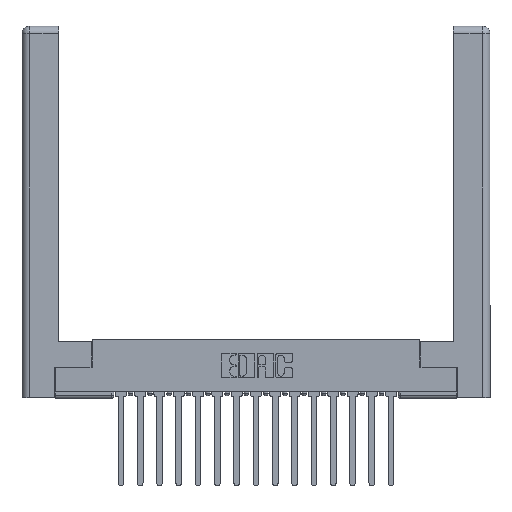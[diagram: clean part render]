
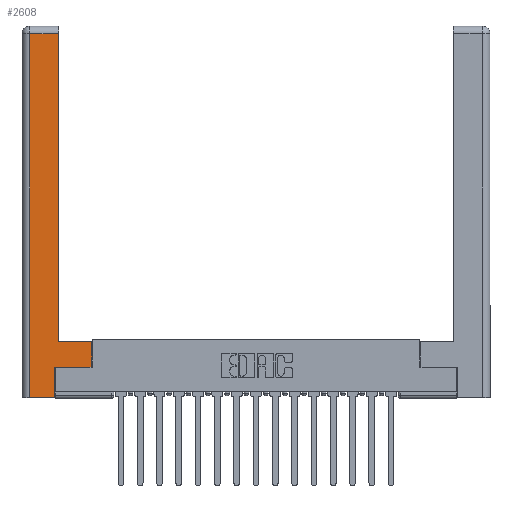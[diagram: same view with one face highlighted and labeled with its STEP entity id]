
A CAD part, top view. The second image highlights one B-rep face of the part: STEP entity #2608.
In plain terms, the highlighted planar face has unit normal (0, 0, 1).
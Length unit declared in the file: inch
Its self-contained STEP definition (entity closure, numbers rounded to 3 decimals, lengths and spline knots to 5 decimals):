
#690 = EDGE_CURVE ( 'NONE', #15175, #12011, #10339, .T. ) ;
#1031 = CARTESIAN_POINT ( 'NONE',  ( 0.565, 0.245, 0. ) ) ;
#1948 = EDGE_CURVE ( 'NONE', #12144, #15175, #2105, .T. ) ;
#2105 = LINE ( 'NONE', #5630, #14569 ) ;
#2279 = EDGE_CURVE ( 'NONE', #12354, #12144, #8084, .T. ) ;
#2391 = LINE ( 'NONE', #11742, #4195 ) ;
#2605 = LINE ( 'NONE', #14823, #12812 ) ;
#2608 = ADVANCED_FACE ( 'NONE', ( #17545 ), #12917, .F. ) ;
#2636 = ORIENTED_EDGE ( 'NONE', *, *, #5507, .T. ) ;
#2843 = DIRECTION ( 'NONE',  ( 0., 1., 0. ) ) ;
#3435 = ORIENTED_EDGE ( 'NONE', *, *, #9175, .T. ) ;
#3594 = CARTESIAN_POINT ( 'NONE',  ( 0.565, 0.45, 0. ) ) ;
#3981 = CARTESIAN_POINT ( 'NONE',  ( 0.295, 0.45, 0. ) ) ;
#4195 = VECTOR ( 'NONE', #17581, 39.37008 ) ;
#4215 = VECTOR ( 'NONE', #10608, 39.37008 ) ;
#4521 = VERTEX_POINT ( 'NONE', #7517 ) ;
#4975 = AXIS2_PLACEMENT_3D ( 'NONE', #14380, #15795, #7072 ) ;
#5380 = VECTOR ( 'NONE', #2843, 39.37008 ) ;
#5507 = EDGE_CURVE ( 'NONE', #13913, #12354, #7568, .T. ) ;
#5630 = CARTESIAN_POINT ( 'NONE',  ( 0.0615, 0., 0. ) ) ;
#6068 = EDGE_CURVE ( 'NONE', #8814, #13913, #10950, .T. ) ;
#6101 = CARTESIAN_POINT ( 'NONE',  ( 0.0615, 0., 0. ) ) ;
#6531 = ORIENTED_EDGE ( 'NONE', *, *, #2279, .T. ) ;
#6798 = VERTEX_POINT ( 'NONE', #1031 ) ;
#7072 = DIRECTION ( 'NONE',  ( -1., 0., 0. ) ) ;
#7517 = CARTESIAN_POINT ( 'NONE',  ( 0.265, 0.245, 0. ) ) ;
#7568 = LINE ( 'NONE', #8309, #16883 ) ;
#7803 = CARTESIAN_POINT ( 'NONE',  ( 0.0615, 2.94, 0. ) ) ;
#8084 = LINE ( 'NONE', #7803, #4215 ) ;
#8309 = CARTESIAN_POINT ( 'NONE',  ( 0.295, 3., 0. ) ) ;
#8814 = VERTEX_POINT ( 'NONE', #3594 ) ;
#9175 = EDGE_CURVE ( 'NONE', #6798, #8814, #14263, .T. ) ;
#9369 = VECTOR ( 'NONE', #13942, 39.37008 ) ;
#9611 = ORIENTED_EDGE ( 'NONE', *, *, #12379, .T. ) ;
#9709 = DIRECTION ( 'NONE',  ( 0., 1., 0. ) ) ;
#10092 = CARTESIAN_POINT ( 'NONE',  ( 0.565, 0.45, 0. ) ) ;
#10339 = LINE ( 'NONE', #14136, #16454 ) ;
#10608 = DIRECTION ( 'NONE',  ( -1., 0., 0. ) ) ;
#10950 = LINE ( 'NONE', #3981, #9369 ) ;
#11403 = ORIENTED_EDGE ( 'NONE', *, *, #1948, .T. ) ;
#11567 = ORIENTED_EDGE ( 'NONE', *, *, #690, .T. ) ;
#11742 = CARTESIAN_POINT ( 'NONE',  ( 0.565, 0.245, 0. ) ) ;
#12011 = VERTEX_POINT ( 'NONE', #13886 ) ;
#12144 = VERTEX_POINT ( 'NONE', #17047 ) ;
#12301 = EDGE_LOOP ( 'NONE', ( #2636, #6531, #11403, #11567, #9611, #17929, #3435, #14772 ) ) ;
#12354 = VERTEX_POINT ( 'NONE', #17652 ) ;
#12379 = EDGE_CURVE ( 'NONE', #12011, #4521, #2605, .T. ) ;
#12812 = VECTOR ( 'NONE', #13181, 39.37008 ) ;
#12917 = PLANE ( 'NONE',  #4975 ) ;
#13181 = DIRECTION ( 'NONE',  ( 0., 1., 0. ) ) ;
#13299 = CARTESIAN_POINT ( 'NONE',  ( 0.295, 0.45, 0. ) ) ;
#13886 = CARTESIAN_POINT ( 'NONE',  ( 0.265, 0., 0. ) ) ;
#13913 = VERTEX_POINT ( 'NONE', #13299 ) ;
#13942 = DIRECTION ( 'NONE',  ( -1., 0., 0. ) ) ;
#14136 = CARTESIAN_POINT ( 'NONE',  ( 0.265, 0., 0. ) ) ;
#14263 = LINE ( 'NONE', #10092, #5380 ) ;
#14380 = CARTESIAN_POINT ( 'NONE',  ( 0., 0., 0. ) ) ;
#14569 = VECTOR ( 'NONE', #18696, 39.37008 ) ;
#14772 = ORIENTED_EDGE ( 'NONE', *, *, #6068, .T. ) ;
#14823 = CARTESIAN_POINT ( 'NONE',  ( 0.265, 0.245, 0. ) ) ;
#15175 = VERTEX_POINT ( 'NONE', #6101 ) ;
#15662 = EDGE_CURVE ( 'NONE', #4521, #6798, #2391, .T. ) ;
#15795 = DIRECTION ( 'NONE',  ( 0., 0., -1. ) ) ;
#16454 = VECTOR ( 'NONE', #16790, 39.37008 ) ;
#16790 = DIRECTION ( 'NONE',  ( 1., 0., 0. ) ) ;
#16883 = VECTOR ( 'NONE', #9709, 39.37008 ) ;
#17047 = CARTESIAN_POINT ( 'NONE',  ( 0.0615, 2.94, 0. ) ) ;
#17545 = FACE_OUTER_BOUND ( 'NONE', #12301, .T. ) ;
#17581 = DIRECTION ( 'NONE',  ( 1., 0., 0. ) ) ;
#17652 = CARTESIAN_POINT ( 'NONE',  ( 0.295, 2.94, 0. ) ) ;
#17929 = ORIENTED_EDGE ( 'NONE', *, *, #15662, .T. ) ;
#18696 = DIRECTION ( 'NONE',  ( 0., -1., 0. ) ) ;
